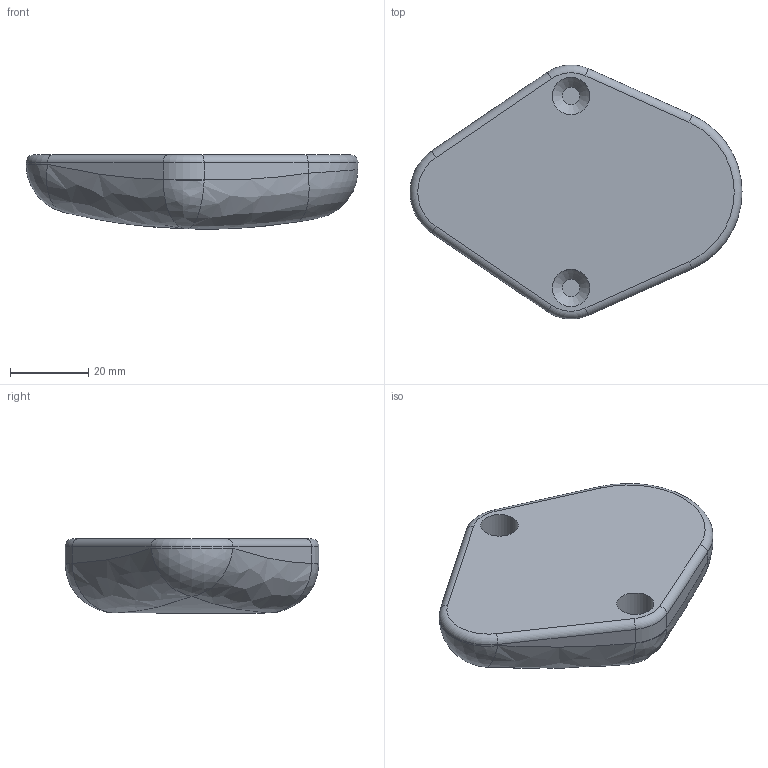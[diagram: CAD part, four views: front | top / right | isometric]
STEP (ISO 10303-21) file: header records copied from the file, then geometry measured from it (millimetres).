
FILE_DESCRIPTION (( 'STEP AP214' ), '1' );
FILE_NAME ('Butt Plate.STEP', '2014-02-12T12:48:34', ( 'elpi' ), ( '' ), 'SwSTEP 2.0', 'SolidWorks 2013', '' );
FILE_SCHEMA (( 'AUTOMOTIVE_DESIGN' ));
Length unit declared in the file: inch
Products named in the file (1): Butt Plate
Bounding box: 85.09 x 65.05 x 19.02 mm (x, y, z)
Volume: 57538.1 mm3; surface area: 10557.5 mm2
Topology: 1 solids, 1 shells, 34 faces, 73 edges, 41 vertices
Faces by surface type: cylinder 11, bspline 9, plane 7, torus 4, cone 2, sphere 1
Full cylindrical faces by diameter (mm): 9.55 x2
Entity records: 1373 total; most frequent: CARTESIAN_POINT 696, DIRECTION 130, ORIENTED_EDGE 130, EDGE_CURVE 65, AXIS2_PLACEMENT_3D 57, EDGE_LOOP 40, VERTEX_POINT 39, FACE_OUTER_BOUND 36
